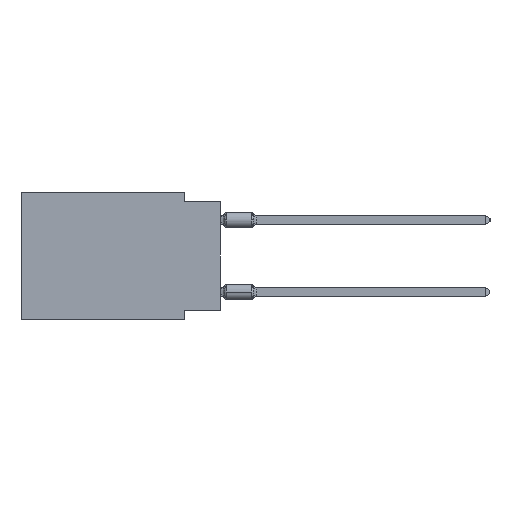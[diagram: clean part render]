
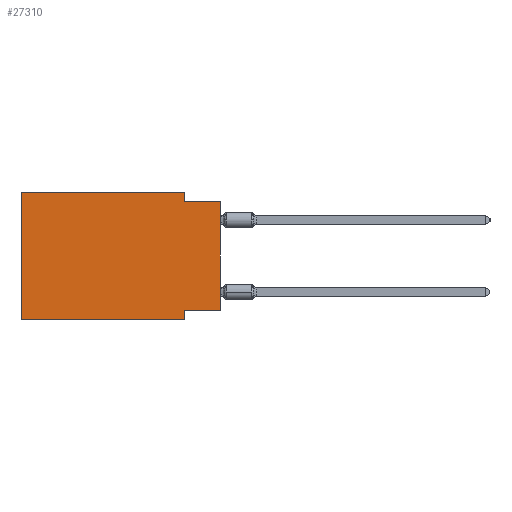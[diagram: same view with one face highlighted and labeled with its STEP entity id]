
A CAD part, left-side view. The second image highlights one B-rep face of the part: STEP entity #27310.
In plain terms, the highlighted planar face has unit normal (-1, 0, 0).
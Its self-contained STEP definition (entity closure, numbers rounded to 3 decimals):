
#920 = DIRECTION ( 'NONE',  ( 0., 0., 1. ) ) ;
#1830 = CARTESIAN_POINT ( 'NONE',  ( 0., 13.97, -8.89 ) ) ;
#2636 = FACE_OUTER_BOUND ( 'NONE', #55124, .T. ) ;
#4776 = VECTOR ( 'NONE', #54505, 1000. ) ;
#6900 = ORIENTED_EDGE ( 'NONE', *, *, #22005, .F. ) ;
#7383 = CARTESIAN_POINT ( 'NONE',  ( 0., 2.54, -0.635 ) ) ;
#7486 = EDGE_CURVE ( 'NONE', #20377, #14983, #41421, .T. ) ;
#7862 = DIRECTION ( 'NONE',  ( 0., 0., -1. ) ) ;
#8377 = EDGE_CURVE ( 'NONE', #61252, #10476, #49332, .T. ) ;
#8761 = CARTESIAN_POINT ( 'NONE',  ( 0., 0., -0.635 ) ) ;
#9124 = CARTESIAN_POINT ( 'NONE',  ( 0., 2.54, 0. ) ) ;
#9335 = CARTESIAN_POINT ( 'NONE',  ( 0., 13.97, 0. ) ) ;
#10228 = DIRECTION ( 'NONE',  ( 0., -1., 0. ) ) ;
#10476 = VERTEX_POINT ( 'NONE', #51052 ) ;
#10485 = VERTEX_POINT ( 'NONE', #17536 ) ;
#10834 = VERTEX_POINT ( 'NONE', #22099 ) ;
#11167 = ORIENTED_EDGE ( 'NONE', *, *, #12448, .T. ) ;
#11343 = LINE ( 'NONE', #1830, #22794 ) ;
#12448 = EDGE_CURVE ( 'NONE', #10485, #10834, #11343, .T. ) ;
#12915 = CARTESIAN_POINT ( 'NONE',  ( 0., 2.54, 0. ) ) ;
#14983 = VERTEX_POINT ( 'NONE', #7383 ) ;
#15003 = LINE ( 'NONE', #29251, #47468 ) ;
#17218 = DIRECTION ( 'NONE',  ( 0., 0., -1. ) ) ;
#17341 = DIRECTION ( 'NONE',  ( 0., -1., 0. ) ) ;
#17536 = CARTESIAN_POINT ( 'NONE',  ( 0., 13.97, -8.89 ) ) ;
#18419 = CARTESIAN_POINT ( 'NONE',  ( 0., 13.97, 0. ) ) ;
#18659 = VECTOR ( 'NONE', #7862, 1000. ) ;
#19017 = EDGE_CURVE ( 'NONE', #45260, #20377, #19730, .T. ) ;
#19323 = LINE ( 'NONE', #18419, #47655 ) ;
#19730 = LINE ( 'NONE', #29549, #20319 ) ;
#20319 = VECTOR ( 'NONE', #10228, 1000. ) ;
#20377 = VERTEX_POINT ( 'NONE', #9124 ) ;
#20833 = AXIS2_PLACEMENT_3D ( 'NONE', #41252, #60541, #17218 ) ;
#21935 = PLANE ( 'NONE',  #20833 ) ;
#22005 = EDGE_CURVE ( 'NONE', #14983, #10476, #60347, .T. ) ;
#22099 = CARTESIAN_POINT ( 'NONE',  ( 0., 2.54, -8.89 ) ) ;
#22794 = VECTOR ( 'NONE', #44897, 1000. ) ;
#27310 = ADVANCED_FACE ( 'NONE', ( #2636 ), #21935, .F. ) ;
#29124 = DIRECTION ( 'NONE',  ( 0., 0., 1. ) ) ;
#29251 = CARTESIAN_POINT ( 'NONE',  ( 0., 0., -8.255 ) ) ;
#29549 = CARTESIAN_POINT ( 'NONE',  ( 0., 13.97, 0. ) ) ;
#29876 = CARTESIAN_POINT ( 'NONE',  ( 0., 2.54, -8.255 ) ) ;
#30112 = ORIENTED_EDGE ( 'NONE', *, *, #7486, .F. ) ;
#31016 = ORIENTED_EDGE ( 'NONE', *, *, #8377, .T. ) ;
#39949 = LINE ( 'NONE', #49427, #4776 ) ;
#40678 = EDGE_CURVE ( 'NONE', #10485, #45260, #19323, .T. ) ;
#41252 = CARTESIAN_POINT ( 'NONE',  ( 0., 13.97, 0. ) ) ;
#41421 = LINE ( 'NONE', #12915, #18659 ) ;
#43494 = DIRECTION ( 'NONE',  ( 0., 1., 0. ) ) ;
#44897 = DIRECTION ( 'NONE',  ( 0., -1., 0. ) ) ;
#45260 = VERTEX_POINT ( 'NONE', #9335 ) ;
#46682 = VECTOR ( 'NONE', #17341, 1000. ) ;
#46872 = ORIENTED_EDGE ( 'NONE', *, *, #19017, .F. ) ;
#47181 = ORIENTED_EDGE ( 'NONE', *, *, #40678, .F. ) ;
#47468 = VECTOR ( 'NONE', #43494, 1000. ) ;
#47655 = VECTOR ( 'NONE', #29124, 1000. ) ;
#48638 = EDGE_CURVE ( 'NONE', #61252, #48708, #15003, .T. ) ;
#48708 = VERTEX_POINT ( 'NONE', #29876 ) ;
#49332 = LINE ( 'NONE', #57904, #50039 ) ;
#49427 = CARTESIAN_POINT ( 'NONE',  ( 0., 2.54, -8.89 ) ) ;
#50039 = VECTOR ( 'NONE', #920, 1000. ) ;
#51052 = CARTESIAN_POINT ( 'NONE',  ( 0., 0., -0.635 ) ) ;
#51139 = EDGE_CURVE ( 'NONE', #48708, #10834, #39949, .T. ) ;
#52986 = CARTESIAN_POINT ( 'NONE',  ( 0., 0., -8.255 ) ) ;
#54505 = DIRECTION ( 'NONE',  ( 0., 0., -1. ) ) ;
#55124 = EDGE_LOOP ( 'NONE', ( #31016, #6900, #30112, #46872, #47181, #11167, #56726, #58647 ) ) ;
#56726 = ORIENTED_EDGE ( 'NONE', *, *, #51139, .F. ) ;
#57904 = CARTESIAN_POINT ( 'NONE',  ( 0., 0., 0. ) ) ;
#58647 = ORIENTED_EDGE ( 'NONE', *, *, #48638, .F. ) ;
#60347 = LINE ( 'NONE', #8761, #46682 ) ;
#60541 = DIRECTION ( 'NONE',  ( 1., 0., 0. ) ) ;
#61252 = VERTEX_POINT ( 'NONE', #52986 ) ;
